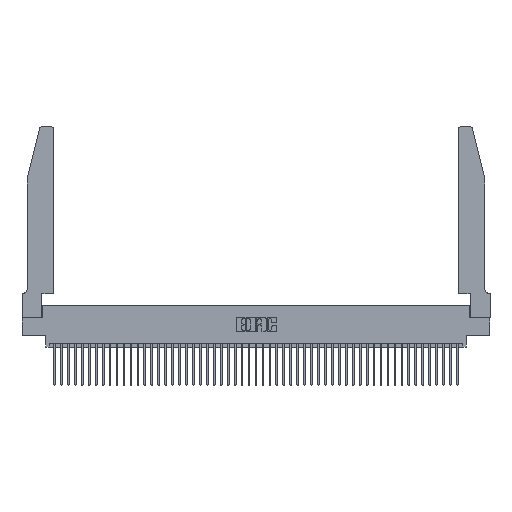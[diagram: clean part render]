
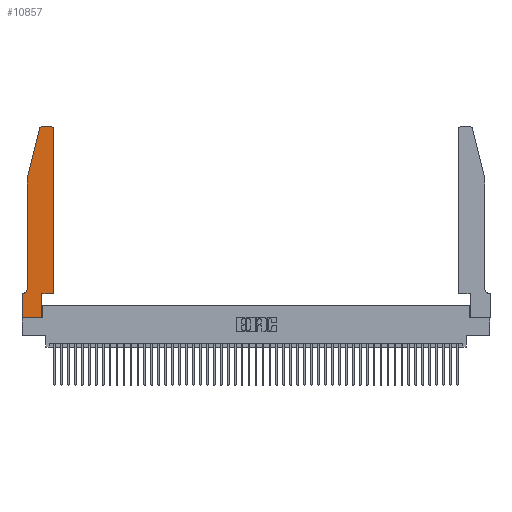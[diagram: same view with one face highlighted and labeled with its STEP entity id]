
A CAD part, top view. The second image highlights one B-rep face of the part: STEP entity #10857.
In plain terms, the highlighted planar face has unit normal (0, 0, 1).
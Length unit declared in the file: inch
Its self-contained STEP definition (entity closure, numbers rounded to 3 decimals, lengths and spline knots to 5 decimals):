
#374 = VECTOR ( 'NONE', #33391, 39.37008 ) ;
#1507 = EDGE_CURVE ( 'NONE', #27866, #39600, #22038, .T. ) ;
#1549 = CIRCLE ( 'NONE', #8127, 0.07 ) ;
#1684 = DIRECTION ( 'NONE',  ( 1., 0., 0. ) ) ;
#1750 = DIRECTION ( 'NONE',  ( 1., 0., 0. ) ) ;
#1787 = EDGE_CURVE ( 'NONE', #40952, #21043, #10789, .T. ) ;
#1795 = VERTEX_POINT ( 'NONE', #44290 ) ;
#2270 = VECTOR ( 'NONE', #43912, 39.37008 ) ;
#2346 = ORIENTED_EDGE ( 'NONE', *, *, #21429, .T. ) ;
#2794 = DIRECTION ( 'NONE',  ( 0., 1., 0. ) ) ;
#3065 = ORIENTED_EDGE ( 'NONE', *, *, #45052, .T. ) ;
#3918 = LINE ( 'NONE', #44814, #374 ) ;
#3995 = VECTOR ( 'NONE', #10950, 39.37008 ) ;
#4120 = VECTOR ( 'NONE', #1684, 39.37008 ) ;
#4188 = DIRECTION ( 'NONE',  ( -1., 0., 0. ) ) ;
#4520 = PLANE ( 'NONE',  #6802 ) ;
#4545 = CARTESIAN_POINT ( 'NONE',  ( 0.4205, 2.75, 0.37 ) ) ;
#6421 = LINE ( 'NONE', #14039, #2270 ) ;
#6802 = AXIS2_PLACEMENT_3D ( 'NONE', #28138, #8352, #47160 ) ;
#8127 = AXIS2_PLACEMENT_3D ( 'NONE', #19284, #26837, #4188 ) ;
#8352 = DIRECTION ( 'NONE',  ( 0., 0., 1. ) ) ;
#10141 = ORIENTED_EDGE ( 'NONE', *, *, #1507, .T. ) ;
#10254 = DIRECTION ( 'NONE',  ( 0., -1., 0. ) ) ;
#10739 = CARTESIAN_POINT ( 'NONE',  ( 0.0755, 2., 0.37 ) ) ;
#10789 = CIRCLE ( 'NONE', #45543, 0.03 ) ;
#10857 = ADVANCED_FACE ( 'NONE', ( #36133 ), #4520, .T. ) ;
#10892 = CARTESIAN_POINT ( 'NONE',  ( 0.0755, 0.42, 0.37 ) ) ;
#10950 = DIRECTION ( 'NONE',  ( 0., -1., 0. ) ) ;
#11143 = VECTOR ( 'NONE', #38534, 39.37008 ) ;
#11258 = ORIENTED_EDGE ( 'NONE', *, *, #16927, .T. ) ;
#11323 = EDGE_CURVE ( 'NONE', #30743, #37475, #1549, .T. ) ;
#12127 = CARTESIAN_POINT ( 'NONE',  ( 0.0755, 0.35, 0.37 ) ) ;
#13472 = DIRECTION ( 'NONE',  ( 0., 0., 1. ) ) ;
#13632 = DIRECTION ( 'NONE',  ( 1., 0., 0. ) ) ;
#14039 = CARTESIAN_POINT ( 'NONE',  ( 0.4505, 0.35, 0.37 ) ) ;
#14180 = CARTESIAN_POINT ( 'NONE',  ( 0.0055, 0.35, 0.37 ) ) ;
#14246 = LINE ( 'NONE', #36079, #4120 ) ;
#14746 = ORIENTED_EDGE ( 'NONE', *, *, #41752, .T. ) ;
#15511 = ORIENTED_EDGE ( 'NONE', *, *, #11323, .T. ) ;
#16927 = EDGE_CURVE ( 'NONE', #37475, #27866, #18273, .T. ) ;
#17946 = DIRECTION ( 'NONE',  ( 0., 0., 1. ) ) ;
#18273 = LINE ( 'NONE', #12127, #11143 ) ;
#19284 = CARTESIAN_POINT ( 'NONE',  ( 0.0055, 0.42, 0.37 ) ) ;
#19595 = CARTESIAN_POINT ( 'NONE',  ( 0., 0., 0.37 ) ) ;
#19650 = CARTESIAN_POINT ( 'NONE',  ( 0.4205, 2.72, 0.37 ) ) ;
#19659 = ORIENTED_EDGE ( 'NONE', *, *, #1787, .T. ) ;
#20164 = VERTEX_POINT ( 'NONE', #26605 ) ;
#20906 = ORIENTED_EDGE ( 'NONE', *, *, #33621, .T. ) ;
#21043 = VERTEX_POINT ( 'NONE', #4545 ) ;
#21429 = EDGE_CURVE ( 'NONE', #42189, #40952, #47617, .T. ) ;
#21929 = EDGE_CURVE ( 'NONE', #1795, #20164, #42818, .T. ) ;
#22038 = LINE ( 'NONE', #43617, #40996 ) ;
#22965 = CARTESIAN_POINT ( 'NONE',  ( 0.284, 2.75, 0.37 ) ) ;
#26605 = CARTESIAN_POINT ( 'NONE',  ( 0.0755, 2., 0.37 ) ) ;
#26837 = DIRECTION ( 'NONE',  ( 0., 0., -1. ) ) ;
#27446 = VECTOR ( 'NONE', #29215, 39.37008 ) ;
#27478 = CARTESIAN_POINT ( 'NONE',  ( 0.2865, 0.35, 0.37 ) ) ;
#27742 = ORIENTED_EDGE ( 'NONE', *, *, #30089, .T. ) ;
#27866 = VERTEX_POINT ( 'NONE', #36185 ) ;
#28138 = CARTESIAN_POINT ( 'NONE',  ( 0., 0.35, 0.37 ) ) ;
#28209 = CIRCLE ( 'NONE', #35012, 0.03 ) ;
#28313 = VECTOR ( 'NONE', #28769, 39.37008 ) ;
#28555 = CARTESIAN_POINT ( 'NONE',  ( 0.4505, 0.35, 0.37 ) ) ;
#28769 = DIRECTION ( 'NONE',  ( -1., 0., 0. ) ) ;
#29110 = CARTESIAN_POINT ( 'NONE',  ( 0.0755, 2., 0.37 ) ) ;
#29215 = DIRECTION ( 'NONE',  ( -0.239, -0.971, 0. ) ) ;
#30089 = EDGE_CURVE ( 'NONE', #41484, #42189, #6421, .T. ) ;
#30743 = VERTEX_POINT ( 'NONE', #10892 ) ;
#31692 = EDGE_CURVE ( 'NONE', #39600, #34304, #14246, .T. ) ;
#32996 = CARTESIAN_POINT ( 'NONE',  ( 0.2865, 0., 0.37 ) ) ;
#32999 = ORIENTED_EDGE ( 'NONE', *, *, #33832, .T. ) ;
#33391 = DIRECTION ( 'NONE',  ( 0., 1., 0. ) ) ;
#33621 = EDGE_CURVE ( 'NONE', #33956, #1795, #28209, .T. ) ;
#33832 = EDGE_CURVE ( 'NONE', #20164, #30743, #40683, .T. ) ;
#33956 = VERTEX_POINT ( 'NONE', #22965 ) ;
#34304 = VERTEX_POINT ( 'NONE', #32996 ) ;
#34558 = VECTOR ( 'NONE', #2794, 39.37008 ) ;
#35012 = AXIS2_PLACEMENT_3D ( 'NONE', #44183, #13472, #13632 ) ;
#36079 = CARTESIAN_POINT ( 'NONE',  ( 0., 0., 0.37 ) ) ;
#36133 = FACE_OUTER_BOUND ( 'NONE', #46709, .T. ) ;
#36185 = CARTESIAN_POINT ( 'NONE',  ( 0., 0.35, 0.37 ) ) ;
#37475 = VERTEX_POINT ( 'NONE', #14180 ) ;
#38534 = DIRECTION ( 'NONE',  ( -1., 0., 0. ) ) ;
#39596 = CARTESIAN_POINT ( 'NONE',  ( 0.4505, 2.72, 0.37 ) ) ;
#39600 = VERTEX_POINT ( 'NONE', #19595 ) ;
#40683 = LINE ( 'NONE', #29110, #3995 ) ;
#40853 = CARTESIAN_POINT ( 'NONE',  ( 0.4505, 0.35, 0.37 ) ) ;
#40952 = VERTEX_POINT ( 'NONE', #39596 ) ;
#40996 = VECTOR ( 'NONE', #10254, 39.37008 ) ;
#41484 = VERTEX_POINT ( 'NONE', #27478 ) ;
#41752 = EDGE_CURVE ( 'NONE', #34304, #41484, #3918, .T. ) ;
#42189 = VERTEX_POINT ( 'NONE', #28555 ) ;
#42818 = LINE ( 'NONE', #10739, #27446 ) ;
#43617 = CARTESIAN_POINT ( 'NONE',  ( 0., 0., 0.37 ) ) ;
#43814 = CARTESIAN_POINT ( 'NONE',  ( 0.2605, 2.75, 0.37 ) ) ;
#43912 = DIRECTION ( 'NONE',  ( 1., 0., 0. ) ) ;
#44183 = CARTESIAN_POINT ( 'NONE',  ( 0.284, 2.72, 0.37 ) ) ;
#44290 = CARTESIAN_POINT ( 'NONE',  ( 0.25487, 2.72718, 0.37 ) ) ;
#44814 = CARTESIAN_POINT ( 'NONE',  ( 0.2865, 0.35, 0.37 ) ) ;
#45052 = EDGE_CURVE ( 'NONE', #21043, #33956, #48424, .T. ) ;
#45543 = AXIS2_PLACEMENT_3D ( 'NONE', #19650, #17946, #1750 ) ;
#46709 = EDGE_LOOP ( 'NONE', ( #3065, #20906, #46828, #32999, #15511, #11258, #10141, #47618, #14746, #27742, #2346, #19659 ) ) ;
#46828 = ORIENTED_EDGE ( 'NONE', *, *, #21929, .T. ) ;
#47160 = DIRECTION ( 'NONE',  ( 1., 0., 0. ) ) ;
#47617 = LINE ( 'NONE', #40853, #34558 ) ;
#47618 = ORIENTED_EDGE ( 'NONE', *, *, #31692, .T. ) ;
#48424 = LINE ( 'NONE', #43814, #28313 ) ;
